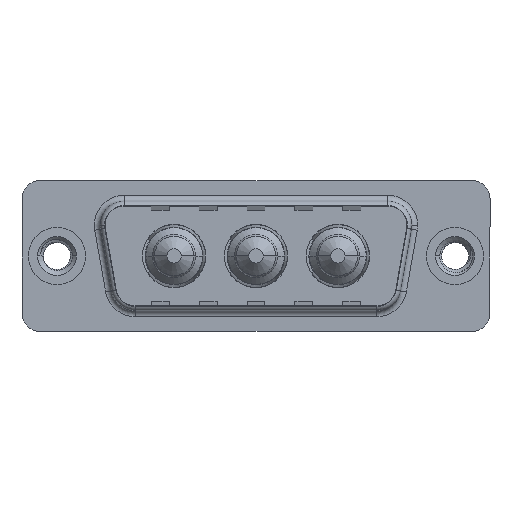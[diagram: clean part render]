
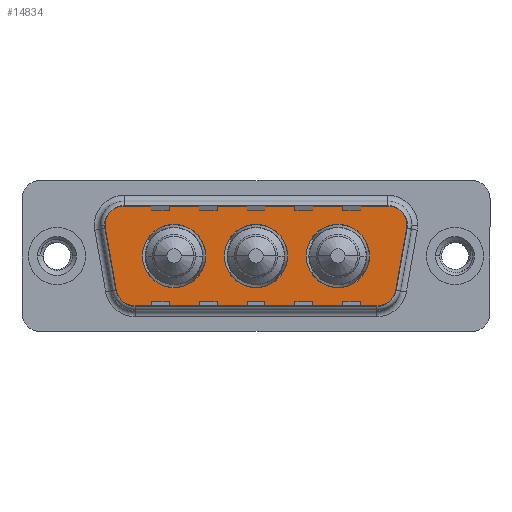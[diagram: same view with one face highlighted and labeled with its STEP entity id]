
A CAD part, top view. The second image highlights one B-rep face of the part: STEP entity #14834.
In plain terms, the highlighted planar face has unit normal (0, 0, 1).
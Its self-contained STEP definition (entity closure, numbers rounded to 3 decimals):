
#46 = EDGE_CURVE ( 'NONE', #2149, #14620, #12160, .T. ) ;
#278 = DIRECTION ( 'NONE',  ( 0., 0., 1. ) ) ;
#356 = AXIS2_PLACEMENT_3D ( 'NONE', #13629, #7463, #7438 ) ;
#429 = EDGE_CURVE ( 'NONE', #10443, #15007, #14860, .T. ) ;
#767 = ORIENTED_EDGE ( 'NONE', *, *, #12464, .T. ) ;
#797 = AXIS2_PLACEMENT_3D ( 'NONE', #12175, #9845, #11236 ) ;
#835 = VECTOR ( 'NONE', #7924, 1000. ) ;
#966 = EDGE_CURVE ( 'NONE', #15007, #5256, #12337, .T. ) ;
#1038 = CIRCLE ( 'NONE', #8767, 2.65 ) ;
#1198 = CIRCLE ( 'NONE', #6889, 2.65 ) ;
#1359 = CARTESIAN_POINT ( 'NONE',  ( 6.434, -4.9, 0. ) ) ;
#1384 = FACE_BOUND ( 'NONE', #9579, .T. ) ;
#1440 = CIRCLE ( 'NONE', #2295, 2. ) ;
#1461 = CARTESIAN_POINT ( 'NONE',  ( 9.8, 0., 0. ) ) ;
#1750 = CARTESIAN_POINT ( 'NONE',  ( 19.3, 0., 0. ) ) ;
#2119 = AXIS2_PLACEMENT_3D ( 'NONE', #14410, #14485, #14700 ) ;
#2149 = VERTEX_POINT ( 'NONE', #1750 ) ;
#2191 = CARTESIAN_POINT ( 'NONE',  ( 3.441, 2.553, 0. ) ) ;
#2271 = CARTESIAN_POINT ( 'NONE',  ( 26.866, -2.9, 0. ) ) ;
#2295 = AXIS2_PLACEMENT_3D ( 'NONE', #9778, #2563, #10999 ) ;
#2317 = DIRECTION ( 'NONE',  ( 0., 0., 1. ) ) ;
#2530 = CARTESIAN_POINT ( 'NONE',  ( 4.464, -3.247, 0. ) ) ;
#2563 = DIRECTION ( 'NONE',  ( 0., 0., 1. ) ) ;
#2664 = DIRECTION ( 'NONE',  ( 1., 0., 0. ) ) ;
#2864 = CARTESIAN_POINT ( 'NONE',  ( 29.859, 2.553, 0. ) ) ;
#3931 = CIRCLE ( 'NONE', #797, 2.65 ) ;
#4182 = EDGE_CURVE ( 'NONE', #14620, #2149, #3931, .T. ) ;
#4270 = CIRCLE ( 'NONE', #356, 2. ) ;
#4291 = VECTOR ( 'NONE', #14601, 1000. ) ;
#4346 = DIRECTION ( 'NONE',  ( 1., 0., 0. ) ) ;
#4417 = CARTESIAN_POINT ( 'NONE',  ( 6.434, -4.9, 0. ) ) ;
#4436 = EDGE_LOOP ( 'NONE', ( #12366, #5808 ) ) ;
#4525 = DIRECTION ( 'NONE',  ( 0.174, 0.985, 0. ) ) ;
#4567 = FACE_BOUND ( 'NONE', #5685, .T. ) ;
#4947 = LINE ( 'NONE', #11838, #14287 ) ;
#5063 = DIRECTION ( 'NONE',  ( 0., 0., 1. ) ) ;
#5256 = VERTEX_POINT ( 'NONE', #15669 ) ;
#5295 = DIRECTION ( 'NONE',  ( 0., 0., 1. ) ) ;
#5363 = CIRCLE ( 'NONE', #8265, 2.65 ) ;
#5418 = EDGE_CURVE ( 'NONE', #6416, #13997, #4270, .T. ) ;
#5482 = CARTESIAN_POINT ( 'NONE',  ( 5.411, 4.9, 0. ) ) ;
#5527 = DIRECTION ( 'NONE',  ( 1., 0., 0. ) ) ;
#5685 = EDGE_LOOP ( 'NONE', ( #13547, #15234 ) ) ;
#5808 = ORIENTED_EDGE ( 'NONE', *, *, #13049, .F. ) ;
#5885 = VECTOR ( 'NONE', #5527, 1000. ) ;
#5913 = VERTEX_POINT ( 'NONE', #6531 ) ;
#5974 = CARTESIAN_POINT ( 'NONE',  ( 5.411, 4.9, 0. ) ) ;
#6098 = CARTESIAN_POINT ( 'NONE',  ( 3.441, 2.553, 0. ) ) ;
#6416 = VERTEX_POINT ( 'NONE', #5974 ) ;
#6466 = VERTEX_POINT ( 'NONE', #12592 ) ;
#6513 = CARTESIAN_POINT ( 'NONE',  ( 23.5, 0., 0. ) ) ;
#6531 = CARTESIAN_POINT ( 'NONE',  ( 7.15, 0., 0. ) ) ;
#6542 = ORIENTED_EDGE ( 'NONE', *, *, #11289, .T. ) ;
#6794 = DIRECTION ( 'NONE',  ( 0., 0., 1. ) ) ;
#6889 = AXIS2_PLACEMENT_3D ( 'NONE', #12327, #5063, #13564 ) ;
#7153 = AXIS2_PLACEMENT_3D ( 'NONE', #1461, #9880, #2664 ) ;
#7301 = VERTEX_POINT ( 'NONE', #12265 ) ;
#7379 = CARTESIAN_POINT ( 'NONE',  ( 12.45, 0., 0. ) ) ;
#7438 = DIRECTION ( 'NONE',  ( 1., 0., 0. ) ) ;
#7463 = DIRECTION ( 'NONE',  ( 0., 0., 1. ) ) ;
#7500 = CIRCLE ( 'NONE', #8542, 2. ) ;
#7527 = CARTESIAN_POINT ( 'NONE',  ( 23.5, 0., 0. ) ) ;
#7769 = AXIS2_PLACEMENT_3D ( 'NONE', #2271, #2317, #10739 ) ;
#7822 = CARTESIAN_POINT ( 'NONE',  ( 27.889, 4.9, 0. ) ) ;
#7924 = DIRECTION ( 'NONE',  ( -1., 0., 0. ) ) ;
#8040 = ORIENTED_EDGE ( 'NONE', *, *, #13057, .F. ) ;
#8241 = EDGE_CURVE ( 'NONE', #9683, #7301, #5363, .T. ) ;
#8265 = AXIS2_PLACEMENT_3D ( 'NONE', #6513, #15021, #4346 ) ;
#8311 = PLANE ( 'NONE',  #7769 ) ;
#8324 = CARTESIAN_POINT ( 'NONE',  ( 20.85, 0., 0. ) ) ;
#8429 = ORIENTED_EDGE ( 'NONE', *, *, #14564, .T. ) ;
#8542 = AXIS2_PLACEMENT_3D ( 'NONE', #12572, #5295, #13832 ) ;
#8674 = EDGE_CURVE ( 'NONE', #10439, #5913, #1198, .T. ) ;
#8730 = DIRECTION ( 'NONE',  ( 1., 0., 0. ) ) ;
#8737 = DIRECTION ( 'NONE',  ( 0., 0., 1. ) ) ;
#8767 = AXIS2_PLACEMENT_3D ( 'NONE', #7527, #278, #8730 ) ;
#8873 = EDGE_CURVE ( 'NONE', #14982, #11559, #15062, .T. ) ;
#9072 = ORIENTED_EDGE ( 'NONE', *, *, #5418, .T. ) ;
#9300 = AXIS2_PLACEMENT_3D ( 'NONE', #14068, #6794, #15286 ) ;
#9500 = EDGE_LOOP ( 'NONE', ( #767, #14919, #13406, #11212, #8429, #9072, #6542, #15281, #14090 ) ) ;
#9563 = EDGE_CURVE ( 'NONE', #6466, #13464, #4947, .T. ) ;
#9579 = EDGE_LOOP ( 'NONE', ( #8040, #13857 ) ) ;
#9683 = VERTEX_POINT ( 'NONE', #8324 ) ;
#9778 = CARTESIAN_POINT ( 'NONE',  ( 27.889, 2.9, 0. ) ) ;
#9845 = DIRECTION ( 'NONE',  ( 0., 0., 1. ) ) ;
#9880 = DIRECTION ( 'NONE',  ( 0., 0., 1. ) ) ;
#10312 = CARTESIAN_POINT ( 'NONE',  ( 16.65, 0., 0. ) ) ;
#10439 = VERTEX_POINT ( 'NONE', #7379 ) ;
#10443 = VERTEX_POINT ( 'NONE', #2530 ) ;
#10446 = LINE ( 'NONE', #5482, #835 ) ;
#10670 = CIRCLE ( 'NONE', #7153, 2.65 ) ;
#10739 = DIRECTION ( 'NONE',  ( 1., 0., 0. ) ) ;
#10960 = CARTESIAN_POINT ( 'NONE',  ( 29.889, 2.9, 0. ) ) ;
#10999 = DIRECTION ( 'NONE',  ( -1., 0., 0. ) ) ;
#11015 = FACE_OUTER_BOUND ( 'NONE', #9500, .T. ) ;
#11212 = ORIENTED_EDGE ( 'NONE', *, *, #8873, .T. ) ;
#11236 = DIRECTION ( 'NONE',  ( 1., 0., 0. ) ) ;
#11289 = EDGE_CURVE ( 'NONE', #13997, #10443, #13612, .T. ) ;
#11396 = FACE_BOUND ( 'NONE', #4436, .T. ) ;
#11559 = VERTEX_POINT ( 'NONE', #7822 ) ;
#11740 = DIRECTION ( 'NONE',  ( 1., 0., 0. ) ) ;
#11838 = CARTESIAN_POINT ( 'NONE',  ( 29.859, 2.553, 0. ) ) ;
#12160 = CIRCLE ( 'NONE', #14920, 2.65 ) ;
#12175 = CARTESIAN_POINT ( 'NONE',  ( 16.65, 0., 0. ) ) ;
#12265 = CARTESIAN_POINT ( 'NONE',  ( 26.15, 0., 0. ) ) ;
#12327 = CARTESIAN_POINT ( 'NONE',  ( 9.8, 0., 0. ) ) ;
#12337 = LINE ( 'NONE', #4417, #5885 ) ;
#12366 = ORIENTED_EDGE ( 'NONE', *, *, #8674, .F. ) ;
#12464 = EDGE_CURVE ( 'NONE', #5256, #6466, #7500, .T. ) ;
#12572 = CARTESIAN_POINT ( 'NONE',  ( 26.866, -2.9, 0. ) ) ;
#12592 = CARTESIAN_POINT ( 'NONE',  ( 28.836, -3.247, 0. ) ) ;
#13005 = EDGE_CURVE ( 'NONE', #13464, #14982, #1440, .T. ) ;
#13049 = EDGE_CURVE ( 'NONE', #5913, #10439, #10670, .T. ) ;
#13057 = EDGE_CURVE ( 'NONE', #7301, #9683, #1038, .T. ) ;
#13406 = ORIENTED_EDGE ( 'NONE', *, *, #13005, .T. ) ;
#13464 = VERTEX_POINT ( 'NONE', #2864 ) ;
#13547 = ORIENTED_EDGE ( 'NONE', *, *, #46, .F. ) ;
#13564 = DIRECTION ( 'NONE',  ( 1., 0., 0. ) ) ;
#13612 = LINE ( 'NONE', #6098, #4291 ) ;
#13629 = CARTESIAN_POINT ( 'NONE',  ( 5.411, 2.9, 0. ) ) ;
#13832 = DIRECTION ( 'NONE',  ( 1., 0., 0. ) ) ;
#13857 = ORIENTED_EDGE ( 'NONE', *, *, #8241, .F. ) ;
#13997 = VERTEX_POINT ( 'NONE', #2191 ) ;
#14068 = CARTESIAN_POINT ( 'NONE',  ( 27.889, 2.9, 0. ) ) ;
#14090 = ORIENTED_EDGE ( 'NONE', *, *, #966, .T. ) ;
#14118 = CARTESIAN_POINT ( 'NONE',  ( 14., 0., 0. ) ) ;
#14287 = VECTOR ( 'NONE', #4525, 1000. ) ;
#14410 = CARTESIAN_POINT ( 'NONE',  ( 6.434, -2.9, 0. ) ) ;
#14485 = DIRECTION ( 'NONE',  ( 0., 0., 1. ) ) ;
#14564 = EDGE_CURVE ( 'NONE', #11559, #6416, #10446, .T. ) ;
#14601 = DIRECTION ( 'NONE',  ( 0.174, -0.985, 0. ) ) ;
#14620 = VERTEX_POINT ( 'NONE', #14118 ) ;
#14700 = DIRECTION ( 'NONE',  ( -1., 0., 0. ) ) ;
#14834 = ADVANCED_FACE ( 'NONE', ( #4567, #1384, #11396, #11015 ), #8311, .T. ) ;
#14860 = CIRCLE ( 'NONE', #2119, 2. ) ;
#14919 = ORIENTED_EDGE ( 'NONE', *, *, #9563, .T. ) ;
#14920 = AXIS2_PLACEMENT_3D ( 'NONE', #10312, #8737, #11740 ) ;
#14982 = VERTEX_POINT ( 'NONE', #10960 ) ;
#15007 = VERTEX_POINT ( 'NONE', #1359 ) ;
#15021 = DIRECTION ( 'NONE',  ( 0., 0., 1. ) ) ;
#15062 = CIRCLE ( 'NONE', #9300, 2. ) ;
#15234 = ORIENTED_EDGE ( 'NONE', *, *, #4182, .F. ) ;
#15281 = ORIENTED_EDGE ( 'NONE', *, *, #429, .T. ) ;
#15286 = DIRECTION ( 'NONE',  ( -1., 0., 0. ) ) ;
#15669 = CARTESIAN_POINT ( 'NONE',  ( 26.866, -4.9, 0. ) ) ;
